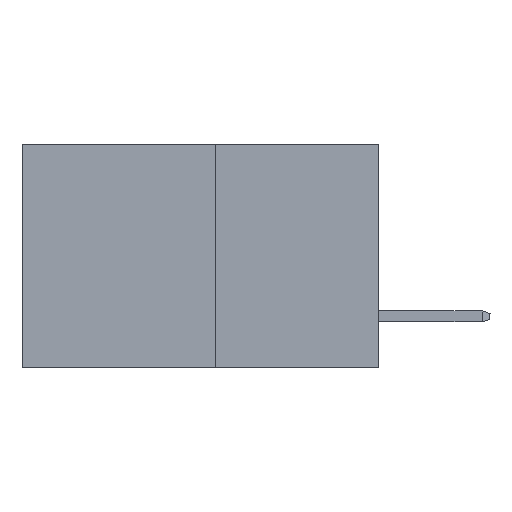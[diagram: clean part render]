
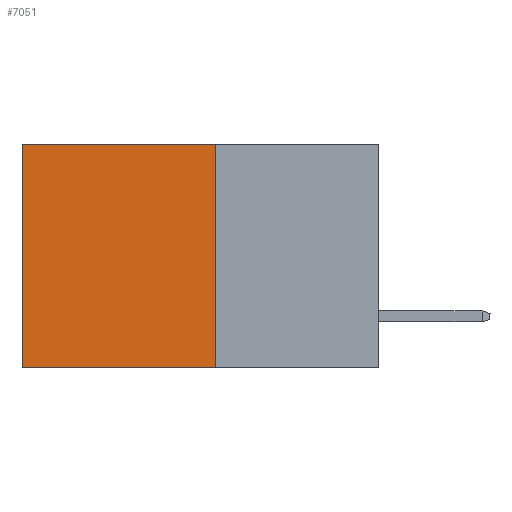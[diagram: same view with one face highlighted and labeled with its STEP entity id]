
A CAD part, left-side view. The second image highlights one B-rep face of the part: STEP entity #7051.
In plain terms, the highlighted planar face has unit normal (-1, 0, 0).
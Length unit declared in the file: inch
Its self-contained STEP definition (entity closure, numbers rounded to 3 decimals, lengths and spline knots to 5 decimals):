
#98 = CARTESIAN_POINT ( 'NONE',  ( 0.277, 0.59, 0. ) ) ;
#109 = AXIS2_PLACEMENT_3D ( 'NONE', #792, #5716, #1519 ) ;
#693 = VECTOR ( 'NONE', #8546, 39.37008 ) ;
#785 = EDGE_CURVE ( 'NONE', #1989, #7173, #6475, .T. ) ;
#792 = CARTESIAN_POINT ( 'NONE',  ( 0.277, 0.27, -0.37 ) ) ;
#1088 = EDGE_CURVE ( 'NONE', #2591, #7173, #6469, .T. ) ;
#1228 = CARTESIAN_POINT ( 'NONE',  ( 0.277, 0.27, -0.37 ) ) ;
#1381 = CARTESIAN_POINT ( 'NONE',  ( 0.277, 0.27, 0. ) ) ;
#1500 = DIRECTION ( 'NONE',  ( 0., 1., 0. ) ) ;
#1519 = DIRECTION ( 'NONE',  ( 0., 0., -1. ) ) ;
#1533 = CARTESIAN_POINT ( 'NONE',  ( 0.277, 0.27, -0.37 ) ) ;
#1548 = EDGE_CURVE ( 'NONE', #8251, #1989, #4469, .T. ) ;
#1989 = VERTEX_POINT ( 'NONE', #98 ) ;
#2222 = DIRECTION ( 'NONE',  ( 0., 1., 0. ) ) ;
#2397 = CARTESIAN_POINT ( 'NONE',  ( 0.277, 0.59, -0.37 ) ) ;
#2591 = VERTEX_POINT ( 'NONE', #6873 ) ;
#2798 = ORIENTED_EDGE ( 'NONE', *, *, #1548, .T. ) ;
#2891 = CARTESIAN_POINT ( 'NONE',  ( 0.277, 0.27, 0. ) ) ;
#2895 = LINE ( 'NONE', #1228, #8098 ) ;
#2909 = PLANE ( 'NONE',  #109 ) ;
#3961 = CARTESIAN_POINT ( 'NONE',  ( 0.277, 0.59, -0.37 ) ) ;
#4240 = ORIENTED_EDGE ( 'NONE', *, *, #1088, .F. ) ;
#4469 = LINE ( 'NONE', #2891, #7582 ) ;
#4530 = EDGE_LOOP ( 'NONE', ( #5857, #4240, #7810, #2798 ) ) ;
#4700 = VECTOR ( 'NONE', #1500, 39.37008 ) ;
#5109 = FACE_OUTER_BOUND ( 'NONE', #4530, .T. ) ;
#5716 = DIRECTION ( 'NONE',  ( 1., 0., 0. ) ) ;
#5857 = ORIENTED_EDGE ( 'NONE', *, *, #785, .T. ) ;
#6469 = LINE ( 'NONE', #1533, #4700 ) ;
#6475 = LINE ( 'NONE', #3961, #693 ) ;
#6873 = CARTESIAN_POINT ( 'NONE',  ( 0.277, 0.27, -0.37 ) ) ;
#7051 = ADVANCED_FACE ( 'NONE', ( #5109 ), #2909, .F. ) ;
#7173 = VERTEX_POINT ( 'NONE', #2397 ) ;
#7396 = EDGE_CURVE ( 'NONE', #8251, #2591, #2895, .T. ) ;
#7582 = VECTOR ( 'NONE', #2222, 39.37008 ) ;
#7810 = ORIENTED_EDGE ( 'NONE', *, *, #7396, .F. ) ;
#8098 = VECTOR ( 'NONE', #8731, 39.37008 ) ;
#8251 = VERTEX_POINT ( 'NONE', #1381 ) ;
#8546 = DIRECTION ( 'NONE',  ( 0., 0., -1. ) ) ;
#8731 = DIRECTION ( 'NONE',  ( 0., 0., -1. ) ) ;
